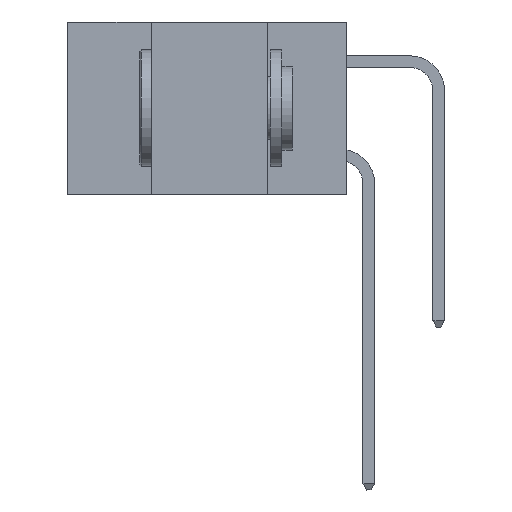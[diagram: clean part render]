
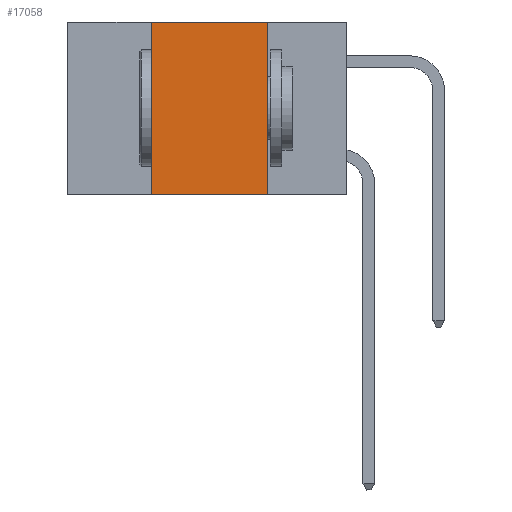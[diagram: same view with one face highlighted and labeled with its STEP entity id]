
A CAD part, left-side view. The second image highlights one B-rep face of the part: STEP entity #17058.
In plain terms, the highlighted planar face has unit normal (-1, 0, 0).
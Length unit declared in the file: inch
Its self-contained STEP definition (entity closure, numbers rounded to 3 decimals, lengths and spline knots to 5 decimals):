
#788 = VECTOR ( 'NONE', #22464, 39.37008 ) ;
#815 = EDGE_CURVE ( 'NONE', #4116, #24897, #17256, .T. ) ;
#875 = DIRECTION ( 'NONE',  ( 1., 0., 0. ) ) ;
#1880 = ORIENTED_EDGE ( 'NONE', *, *, #13967, .F. ) ;
#2329 = CARTESIAN_POINT ( 'NONE',  ( 0., 0.17, 0. ) ) ;
#3366 = CARTESIAN_POINT ( 'NONE',  ( 0., 0.17, -0.37 ) ) ;
#4116 = VERTEX_POINT ( 'NONE', #21066 ) ;
#4672 = VECTOR ( 'NONE', #26937, 39.37008 ) ;
#4920 = CARTESIAN_POINT ( 'NONE',  ( 0., 0.6, -0.37 ) ) ;
#5739 = CARTESIAN_POINT ( 'NONE',  ( 0., 0.17, 0. ) ) ;
#7073 = CARTESIAN_POINT ( 'NONE',  ( 0., 0.6, 0. ) ) ;
#8115 = ORIENTED_EDGE ( 'NONE', *, *, #18405, .F. ) ;
#9342 = EDGE_LOOP ( 'NONE', ( #12511, #8115, #1880, #19468 ) ) ;
#9823 = LINE ( 'NONE', #2329, #16650 ) ;
#12182 = PLANE ( 'NONE',  #19089 ) ;
#12501 = CARTESIAN_POINT ( 'NONE',  ( 0., 0.6, 0. ) ) ;
#12511 = ORIENTED_EDGE ( 'NONE', *, *, #13191, .F. ) ;
#12896 = LINE ( 'NONE', #29690, #13656 ) ;
#13191 = EDGE_CURVE ( 'NONE', #30868, #24897, #9823, .T. ) ;
#13656 = VECTOR ( 'NONE', #19612, 39.37008 ) ;
#13753 = LINE ( 'NONE', #12501, #788 ) ;
#13967 = EDGE_CURVE ( 'NONE', #4116, #26122, #12896, .T. ) ;
#16650 = VECTOR ( 'NONE', #16921, 39.37008 ) ;
#16921 = DIRECTION ( 'NONE',  ( 0., 0., -1. ) ) ;
#17058 = ADVANCED_FACE ( 'NONE', ( #18784 ), #12182, .F. ) ;
#17256 = LINE ( 'NONE', #4920, #4672 ) ;
#18405 = EDGE_CURVE ( 'NONE', #26122, #30868, #13753, .T. ) ;
#18784 = FACE_OUTER_BOUND ( 'NONE', #9342, .T. ) ;
#19089 = AXIS2_PLACEMENT_3D ( 'NONE', #7073, #875, #23293 ) ;
#19468 = ORIENTED_EDGE ( 'NONE', *, *, #815, .T. ) ;
#19612 = DIRECTION ( 'NONE',  ( 0., 0., 1. ) ) ;
#20315 = CARTESIAN_POINT ( 'NONE',  ( 0., 0.42, 0. ) ) ;
#21066 = CARTESIAN_POINT ( 'NONE',  ( 0., 0.42, -0.37 ) ) ;
#22464 = DIRECTION ( 'NONE',  ( 0., -1., 0. ) ) ;
#23293 = DIRECTION ( 'NONE',  ( 0., 0., -1. ) ) ;
#24897 = VERTEX_POINT ( 'NONE', #3366 ) ;
#26122 = VERTEX_POINT ( 'NONE', #20315 ) ;
#26937 = DIRECTION ( 'NONE',  ( 0., -1., 0. ) ) ;
#29690 = CARTESIAN_POINT ( 'NONE',  ( 0., 0.42, 0. ) ) ;
#30868 = VERTEX_POINT ( 'NONE', #5739 ) ;
